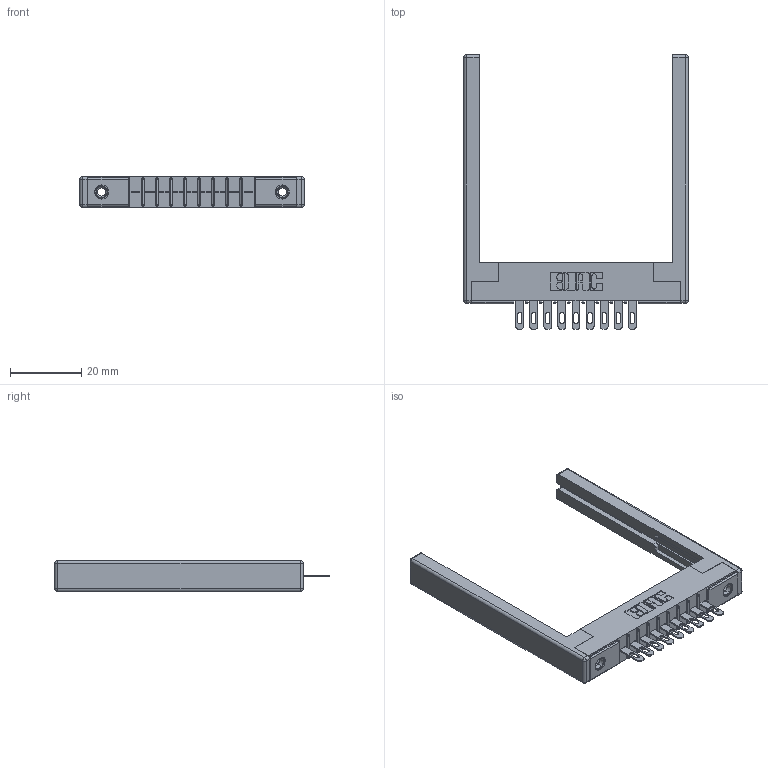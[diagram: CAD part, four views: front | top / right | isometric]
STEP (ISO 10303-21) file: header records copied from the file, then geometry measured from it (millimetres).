
FILE_DESCRIPTION (( 'STEP AP203' ), '1' );
FILE_NAME ('306-009-400-168.STEP', '2020-09-21T15:56:41', ( '' ), ( '' ), 'SwSTEP 2.0', 'SolidWorks 2020', '' );
FILE_SCHEMA (( 'CONFIG_CONTROL_DESIGN' ));
Length unit declared in the file: inch
Products named in the file (5): 306 Part_.156 Dia; 306-009-400-168; 307-220-068; 306-290-001_100; 345-250-001_345-250-001-102
Assembly tree (14 placements, depth 2):
  306-009-400-168
    306 Part_.156 Dia
    306-290-001_100  x9
    345-250-001_345-250-001-102  x2
    307-220-068  x2
Bounding box: 63.09 x 77.17 x 8.71 mm (x, y, z)
Volume: 8831 mm3; surface area: 10187.5 mm2
Topology: 14 solids, 14 shells, 954 faces, 2641 edges, 1690 vertices
Faces by surface type: plane 606, cylinder 288, sphere 44, cone 12, torus 4
Entity records: 15591 total; most frequent: CARTESIAN_POINT 2579, DIRECTION 2560, ORIENTED_EDGE 2544, EDGE_CURVE 1272, VECTOR 970, LINE 970, VERTEX_POINT 814, AXIS2_PLACEMENT_3D 795
